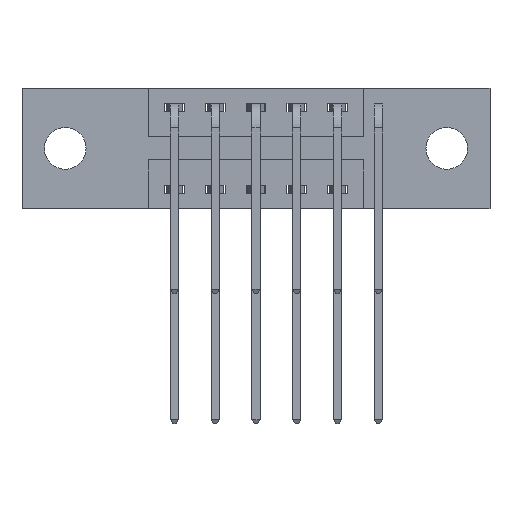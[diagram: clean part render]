
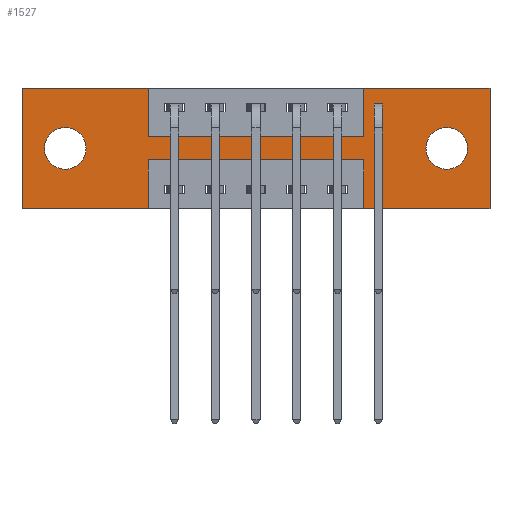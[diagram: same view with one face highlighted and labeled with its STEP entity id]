
A CAD part, front view. The second image highlights one B-rep face of the part: STEP entity #1527.
In plain terms, the highlighted planar face has unit normal (0, -1, 0).
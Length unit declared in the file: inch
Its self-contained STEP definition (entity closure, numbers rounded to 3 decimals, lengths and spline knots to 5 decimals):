
#10 = DIRECTION ( 'NONE',  ( 0., 0., 1. ) ) ;
#84 = DIRECTION ( 'NONE',  ( 0., 1., 0. ) ) ;
#205 = DIRECTION ( 'NONE',  ( 0., 0., 1. ) ) ;
#211 = CARTESIAN_POINT ( 'NONE',  ( 0.1325, 0., -0.185 ) ) ;
#254 = CARTESIAN_POINT ( 'NONE',  ( 1.435, 0., 0. ) ) ;
#399 = VECTOR ( 'NONE', #2186, 39.37008 ) ;
#513 = CARTESIAN_POINT ( 'NONE',  ( 1.0475, 0., 0. ) ) ;
#582 = VERTEX_POINT ( 'NONE', #6050 ) ;
#733 = VECTOR ( 'NONE', #7360, 39.37008 ) ;
#823 = CARTESIAN_POINT ( 'NONE',  ( 1.0475, 0., -0.15 ) ) ;
#840 = CARTESIAN_POINT ( 'NONE',  ( 1.435, 0., -0.37 ) ) ;
#1117 = ORIENTED_EDGE ( 'NONE', *, *, #3911, .F. ) ;
#1198 = PLANE ( 'NONE',  #4856 ) ;
#1251 = FACE_OUTER_BOUND ( 'NONE', #4198, .T. ) ;
#1252 = CARTESIAN_POINT ( 'NONE',  ( 0.3875, 0., -0.37 ) ) ;
#1273 = VERTEX_POINT ( 'NONE', #2335 ) ;
#1306 = CARTESIAN_POINT ( 'NONE',  ( 0., 0., -0.37 ) ) ;
#1307 = DIRECTION ( 'NONE',  ( 0., 0., -1. ) ) ;
#1365 = CARTESIAN_POINT ( 'NONE',  ( 1.3025, 0., -0.185 ) ) ;
#1377 = EDGE_CURVE ( 'NONE', #9402, #2060, #2680, .T. ) ;
#1415 = VECTOR ( 'NONE', #8904, 39.37008 ) ;
#1430 = ORIENTED_EDGE ( 'NONE', *, *, #4567, .F. ) ;
#1527 = ADVANCED_FACE ( 'NONE', ( #5813, #6782, #1251 ), #1198, .T. ) ;
#1661 = EDGE_CURVE ( 'NONE', #9852, #9010, #7654, .T. ) ;
#1678 = CARTESIAN_POINT ( 'NONE',  ( 0.3875, 0., -0.22 ) ) ;
#1760 = EDGE_CURVE ( 'NONE', #9457, #9072, #5306, .T. ) ;
#2047 = CIRCLE ( 'NONE', #3701, 0.064 ) ;
#2055 = ORIENTED_EDGE ( 'NONE', *, *, #7052, .F. ) ;
#2060 = VERTEX_POINT ( 'NONE', #1678 ) ;
#2184 = DIRECTION ( 'NONE',  ( 0., 1., 0. ) ) ;
#2186 = DIRECTION ( 'NONE',  ( 0., 0., 1. ) ) ;
#2335 = CARTESIAN_POINT ( 'NONE',  ( 0.3875, 0., -0.37 ) ) ;
#2588 = CARTESIAN_POINT ( 'NONE',  ( 0.1325, 0., -0.185 ) ) ;
#2627 = LINE ( 'NONE', #5759, #1415 ) ;
#2670 = DIRECTION ( 'NONE',  ( 1., 0., 0. ) ) ;
#2680 = LINE ( 'NONE', #4170, #733 ) ;
#2720 = CARTESIAN_POINT ( 'NONE',  ( 0., 0., 0. ) ) ;
#2723 = EDGE_CURVE ( 'NONE', #6556, #582, #2047, .T. ) ;
#2985 = CARTESIAN_POINT ( 'NONE',  ( 0., 0., -0.37 ) ) ;
#3175 = EDGE_CURVE ( 'NONE', #1273, #9817, #2627, .T. ) ;
#3186 = EDGE_CURVE ( 'NONE', #3618, #7668, #3442, .T. ) ;
#3274 = VERTEX_POINT ( 'NONE', #9895 ) ;
#3385 = DIRECTION ( 'NONE',  ( 1., 0., 0. ) ) ;
#3442 = LINE ( 'NONE', #9682, #7465 ) ;
#3517 = CARTESIAN_POINT ( 'NONE',  ( 0.1325, 0., -0.121 ) ) ;
#3618 = VERTEX_POINT ( 'NONE', #5790 ) ;
#3701 = AXIS2_PLACEMENT_3D ( 'NONE', #2588, #6400, #4173 ) ;
#3702 = VECTOR ( 'NONE', #6892, 39.37008 ) ;
#3723 = AXIS2_PLACEMENT_3D ( 'NONE', #5521, #84, #5410 ) ;
#3858 = CARTESIAN_POINT ( 'NONE',  ( 0., 0., 0. ) ) ;
#3911 = EDGE_CURVE ( 'NONE', #9072, #9402, #6317, .T. ) ;
#4170 = CARTESIAN_POINT ( 'NONE',  ( 0.3875, 0., -0.22 ) ) ;
#4173 = DIRECTION ( 'NONE',  ( 0., 0., 1. ) ) ;
#4198 = EDGE_LOOP ( 'NONE', ( #2055, #6898, #1117, #8880, #7211, #6167, #5188, #4985, #1430, #6913, #9646, #9913 ) ) ;
#4206 = EDGE_CURVE ( 'NONE', #3274, #5874, #8113, .T. ) ;
#4432 = VECTOR ( 'NONE', #1307, 39.37008 ) ;
#4477 = DIRECTION ( 'NONE',  ( 0., -1., 0. ) ) ;
#4522 = VERTEX_POINT ( 'NONE', #6113 ) ;
#4567 = EDGE_CURVE ( 'NONE', #9010, #3618, #9222, .T. ) ;
#4612 = LINE ( 'NONE', #3858, #8010 ) ;
#4788 = EDGE_CURVE ( 'NONE', #582, #6556, #9452, .T. ) ;
#4856 = AXIS2_PLACEMENT_3D ( 'NONE', #1306, #4477, #7601 ) ;
#4985 = ORIENTED_EDGE ( 'NONE', *, *, #3186, .F. ) ;
#5019 = LINE ( 'NONE', #254, #8497 ) ;
#5028 = VERTEX_POINT ( 'NONE', #9102 ) ;
#5188 = ORIENTED_EDGE ( 'NONE', *, *, #7879, .F. ) ;
#5306 = LINE ( 'NONE', #2985, #9243 ) ;
#5410 = DIRECTION ( 'NONE',  ( 0., 0., -1. ) ) ;
#5421 = LINE ( 'NONE', #513, #399 ) ;
#5521 = CARTESIAN_POINT ( 'NONE',  ( 1.3025, 0., -0.185 ) ) ;
#5590 = AXIS2_PLACEMENT_3D ( 'NONE', #1365, #2184, #7665 ) ;
#5759 = CARTESIAN_POINT ( 'NONE',  ( 0., 0., -0.37 ) ) ;
#5790 = CARTESIAN_POINT ( 'NONE',  ( 0.3875, 0., -0.15 ) ) ;
#5813 = FACE_BOUND ( 'NONE', #6961, .T. ) ;
#5874 = VERTEX_POINT ( 'NONE', #6172 ) ;
#6050 = CARTESIAN_POINT ( 'NONE',  ( 0.1325, 0., -0.249 ) ) ;
#6113 = CARTESIAN_POINT ( 'NONE',  ( 1.0475, 0., 0. ) ) ;
#6127 = CARTESIAN_POINT ( 'NONE',  ( 0., 0., 0. ) ) ;
#6143 = ORIENTED_EDGE ( 'NONE', *, *, #4788, .T. ) ;
#6167 = ORIENTED_EDGE ( 'NONE', *, *, #8516, .F. ) ;
#6172 = CARTESIAN_POINT ( 'NONE',  ( 1.3025, 0., -0.121 ) ) ;
#6245 = EDGE_LOOP ( 'NONE', ( #8278, #6143 ) ) ;
#6317 = LINE ( 'NONE', #7824, #7172 ) ;
#6337 = CARTESIAN_POINT ( 'NONE',  ( 1.0475, 0., -0.22 ) ) ;
#6400 = DIRECTION ( 'NONE',  ( 0., 1., 0. ) ) ;
#6518 = EDGE_CURVE ( 'NONE', #5028, #9457, #5019, .T. ) ;
#6556 = VERTEX_POINT ( 'NONE', #3517 ) ;
#6674 = LINE ( 'NONE', #2720, #7579 ) ;
#6756 = EDGE_CURVE ( 'NONE', #5874, #3274, #8644, .T. ) ;
#6782 = FACE_BOUND ( 'NONE', #6245, .T. ) ;
#6892 = DIRECTION ( 'NONE',  ( 1., 0., 0. ) ) ;
#6898 = ORIENTED_EDGE ( 'NONE', *, *, #1377, .F. ) ;
#6913 = ORIENTED_EDGE ( 'NONE', *, *, #1661, .F. ) ;
#6961 = EDGE_LOOP ( 'NONE', ( #9298, #9586 ) ) ;
#7052 = EDGE_CURVE ( 'NONE', #2060, #1273, #9850, .T. ) ;
#7105 = CARTESIAN_POINT ( 'NONE',  ( 1.0475, 0., -0.37 ) ) ;
#7172 = VECTOR ( 'NONE', #205, 39.37008 ) ;
#7211 = ORIENTED_EDGE ( 'NONE', *, *, #6518, .F. ) ;
#7360 = DIRECTION ( 'NONE',  ( -1., 0., 0. ) ) ;
#7435 = CARTESIAN_POINT ( 'NONE',  ( 0., 0., -0.37 ) ) ;
#7465 = VECTOR ( 'NONE', #2670, 39.37008 ) ;
#7579 = VECTOR ( 'NONE', #3385, 39.37008 ) ;
#7601 = DIRECTION ( 'NONE',  ( 0., 0., -1. ) ) ;
#7654 = LINE ( 'NONE', #6127, #3702 ) ;
#7665 = DIRECTION ( 'NONE',  ( 0., 0., -1. ) ) ;
#7668 = VERTEX_POINT ( 'NONE', #823 ) ;
#7807 = AXIS2_PLACEMENT_3D ( 'NONE', #211, #8541, #7980 ) ;
#7824 = CARTESIAN_POINT ( 'NONE',  ( 1.0475, 0., -0.37 ) ) ;
#7856 = CARTESIAN_POINT ( 'NONE',  ( 0.3875, 0., 0. ) ) ;
#7879 = EDGE_CURVE ( 'NONE', #7668, #4522, #5421, .T. ) ;
#7980 = DIRECTION ( 'NONE',  ( 0., 0., 1. ) ) ;
#8010 = VECTOR ( 'NONE', #10, 39.37008 ) ;
#8020 = DIRECTION ( 'NONE',  ( 0., 0., -1. ) ) ;
#8113 = CIRCLE ( 'NONE', #3723, 0.064 ) ;
#8278 = ORIENTED_EDGE ( 'NONE', *, *, #2723, .T. ) ;
#8401 = DIRECTION ( 'NONE',  ( -1., 0., 0. ) ) ;
#8497 = VECTOR ( 'NONE', #8020, 39.37008 ) ;
#8516 = EDGE_CURVE ( 'NONE', #4522, #5028, #6674, .T. ) ;
#8541 = DIRECTION ( 'NONE',  ( 0., 1., 0. ) ) ;
#8644 = CIRCLE ( 'NONE', #5590, 0.064 ) ;
#8780 = VECTOR ( 'NONE', #9275, 39.37008 ) ;
#8880 = ORIENTED_EDGE ( 'NONE', *, *, #1760, .F. ) ;
#8904 = DIRECTION ( 'NONE',  ( -1., 0., 0. ) ) ;
#9010 = VERTEX_POINT ( 'NONE', #7856 ) ;
#9072 = VERTEX_POINT ( 'NONE', #7105 ) ;
#9102 = CARTESIAN_POINT ( 'NONE',  ( 1.435, 0., 0. ) ) ;
#9115 = CARTESIAN_POINT ( 'NONE',  ( 0.3875, 0., 0. ) ) ;
#9222 = LINE ( 'NONE', #9115, #8780 ) ;
#9243 = VECTOR ( 'NONE', #8401, 39.37008 ) ;
#9275 = DIRECTION ( 'NONE',  ( 0., 0., -1. ) ) ;
#9298 = ORIENTED_EDGE ( 'NONE', *, *, #6756, .T. ) ;
#9402 = VERTEX_POINT ( 'NONE', #6337 ) ;
#9452 = CIRCLE ( 'NONE', #7807, 0.064 ) ;
#9457 = VERTEX_POINT ( 'NONE', #840 ) ;
#9586 = ORIENTED_EDGE ( 'NONE', *, *, #4206, .T. ) ;
#9646 = ORIENTED_EDGE ( 'NONE', *, *, #9946, .F. ) ;
#9682 = CARTESIAN_POINT ( 'NONE',  ( 0.3875, 0., -0.15 ) ) ;
#9817 = VERTEX_POINT ( 'NONE', #7435 ) ;
#9850 = LINE ( 'NONE', #1252, #4432 ) ;
#9852 = VERTEX_POINT ( 'NONE', #10099 ) ;
#9895 = CARTESIAN_POINT ( 'NONE',  ( 1.3025, 0., -0.249 ) ) ;
#9913 = ORIENTED_EDGE ( 'NONE', *, *, #3175, .F. ) ;
#9946 = EDGE_CURVE ( 'NONE', #9817, #9852, #4612, .T. ) ;
#10099 = CARTESIAN_POINT ( 'NONE',  ( 0., 0., 0. ) ) ;
